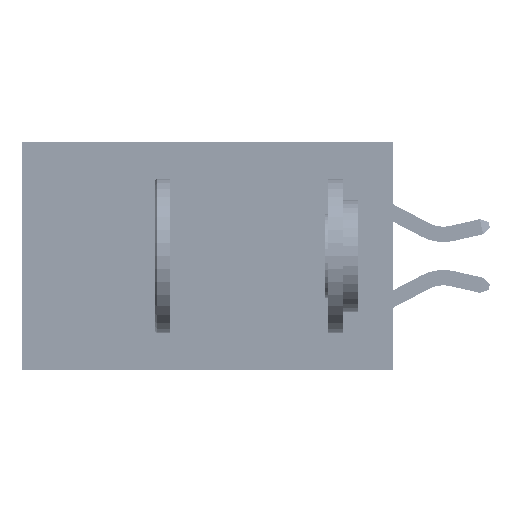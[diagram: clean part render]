
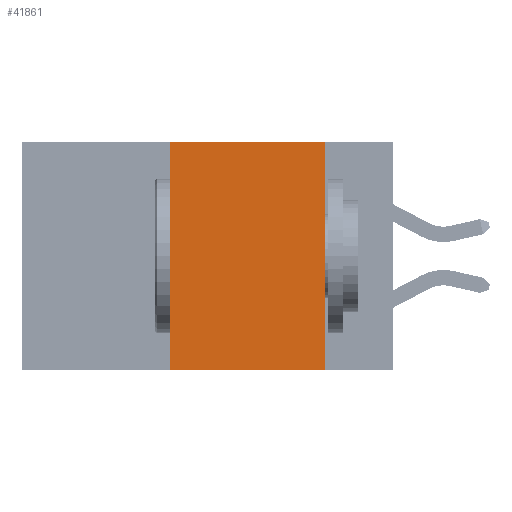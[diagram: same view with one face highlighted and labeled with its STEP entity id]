
A CAD part, left-side view. The second image highlights one B-rep face of the part: STEP entity #41861.
In plain terms, the highlighted planar face has unit normal (-1, 0, 0).
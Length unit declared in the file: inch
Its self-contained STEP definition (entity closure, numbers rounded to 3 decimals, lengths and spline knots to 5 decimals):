
#227 = ORIENTED_EDGE ( 'NONE', *, *, #7520, .T. ) ;
#587 = DIRECTION ( 'NONE',  ( 0., -1., 0. ) ) ;
#893 = EDGE_CURVE ( 'NONE', #39806, #5921, #1890, .T. ) ;
#1890 = LINE ( 'NONE', #49030, #15822 ) ;
#4343 = VERTEX_POINT ( 'NONE', #37655 ) ;
#5650 = CARTESIAN_POINT ( 'NONE',  ( 0., 0.11, -0.37 ) ) ;
#5921 = VERTEX_POINT ( 'NONE', #28795 ) ;
#7204 = VECTOR ( 'NONE', #22635, 39.37008 ) ;
#7520 = EDGE_CURVE ( 'NONE', #39806, #44883, #8912, .T. ) ;
#8912 = LINE ( 'NONE', #12231, #16791 ) ;
#10759 = EDGE_LOOP ( 'NONE', ( #29180, #39686, #34399, #227 ) ) ;
#12231 = CARTESIAN_POINT ( 'NONE',  ( 0., 0.6, -0.37 ) ) ;
#13392 = VECTOR ( 'NONE', #29248, 39.37008 ) ;
#13661 = PLANE ( 'NONE',  #48285 ) ;
#15822 = VECTOR ( 'NONE', #17818, 39.37008 ) ;
#16734 = EDGE_CURVE ( 'NONE', #4343, #44883, #48487, .T. ) ;
#16791 = VECTOR ( 'NONE', #587, 39.37008 ) ;
#17748 = DIRECTION ( 'NONE',  ( 0., 0., -1. ) ) ;
#17818 = DIRECTION ( 'NONE',  ( 0., 0., 1. ) ) ;
#22635 = DIRECTION ( 'NONE',  ( 0., 0., -1. ) ) ;
#25069 = DIRECTION ( 'NONE',  ( 1., 0., 0. ) ) ;
#26313 = FACE_OUTER_BOUND ( 'NONE', #10759, .T. ) ;
#28795 = CARTESIAN_POINT ( 'NONE',  ( 0., 0.36, 0. ) ) ;
#29180 = ORIENTED_EDGE ( 'NONE', *, *, #16734, .F. ) ;
#29248 = DIRECTION ( 'NONE',  ( 0., -1., 0. ) ) ;
#34399 = ORIENTED_EDGE ( 'NONE', *, *, #893, .F. ) ;
#37655 = CARTESIAN_POINT ( 'NONE',  ( 0., 0.11, 0. ) ) ;
#37794 = EDGE_CURVE ( 'NONE', #5921, #4343, #39524, .T. ) ;
#39524 = LINE ( 'NONE', #44709, #13392 ) ;
#39686 = ORIENTED_EDGE ( 'NONE', *, *, #37794, .F. ) ;
#39806 = VERTEX_POINT ( 'NONE', #47365 ) ;
#41861 = ADVANCED_FACE ( 'NONE', ( #26313 ), #13661, .F. ) ;
#44709 = CARTESIAN_POINT ( 'NONE',  ( 0., 0.6, 0. ) ) ;
#44883 = VERTEX_POINT ( 'NONE', #5650 ) ;
#45884 = CARTESIAN_POINT ( 'NONE',  ( 0., 0.11, 0. ) ) ;
#47365 = CARTESIAN_POINT ( 'NONE',  ( 0., 0.36, -0.37 ) ) ;
#48285 = AXIS2_PLACEMENT_3D ( 'NONE', #48967, #25069, #17748 ) ;
#48487 = LINE ( 'NONE', #45884, #7204 ) ;
#48967 = CARTESIAN_POINT ( 'NONE',  ( 0., 0.6, 0. ) ) ;
#49030 = CARTESIAN_POINT ( 'NONE',  ( 0., 0.36, 0. ) ) ;
